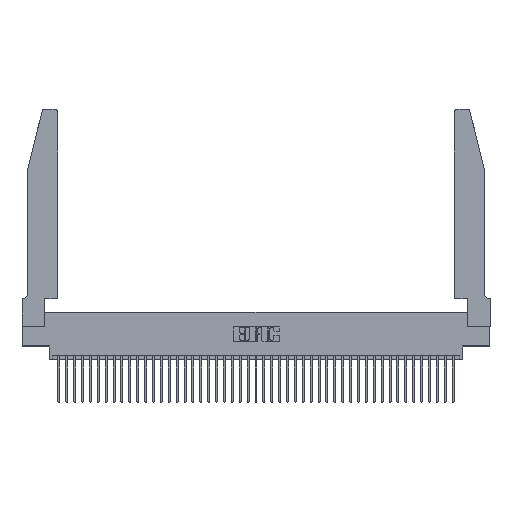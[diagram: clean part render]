
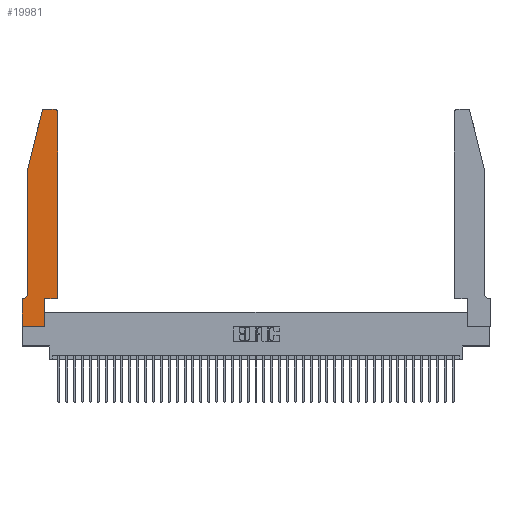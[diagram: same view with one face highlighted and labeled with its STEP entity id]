
A CAD part, top view. The second image highlights one B-rep face of the part: STEP entity #19981.
In plain terms, the highlighted planar face has unit normal (0, 0, 1).
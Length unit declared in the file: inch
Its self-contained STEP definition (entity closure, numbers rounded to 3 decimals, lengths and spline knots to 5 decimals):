
#165 = DIRECTION ( 'NONE',  ( 0., 1., 0. ) ) ;
#178 = CARTESIAN_POINT ( 'NONE',  ( 0.4505, 2.72, 0.37 ) ) ;
#245 = EDGE_CURVE ( 'NONE', #32430, #16549, #14913, .T. ) ;
#599 = ORIENTED_EDGE ( 'NONE', *, *, #18778, .T. ) ;
#636 = AXIS2_PLACEMENT_3D ( 'NONE', #8367, #5128, #24774 ) ;
#675 = DIRECTION ( 'NONE',  ( 1., 0., 0. ) ) ;
#732 = CARTESIAN_POINT ( 'NONE',  ( 0.0755, 2., 0.37 ) ) ;
#1567 = VECTOR ( 'NONE', #165, 39.37008 ) ;
#1759 = VERTEX_POINT ( 'NONE', #36868 ) ;
#1769 = EDGE_CURVE ( 'NONE', #6886, #20490, #16434, .T. ) ;
#1901 = DIRECTION ( 'NONE',  ( 0., -1., 0. ) ) ;
#2114 = DIRECTION ( 'NONE',  ( 1., 0., 0. ) ) ;
#3826 = CARTESIAN_POINT ( 'NONE',  ( 0.284, 2.75, 0.37 ) ) ;
#3864 = ORIENTED_EDGE ( 'NONE', *, *, #32552, .T. ) ;
#4105 = CARTESIAN_POINT ( 'NONE',  ( 0.2865, 0.35, 0.37 ) ) ;
#4147 = AXIS2_PLACEMENT_3D ( 'NONE', #11711, #27292, #17584 ) ;
#4201 = ORIENTED_EDGE ( 'NONE', *, *, #20687, .T. ) ;
#4270 = ORIENTED_EDGE ( 'NONE', *, *, #27838, .T. ) ;
#4411 = CIRCLE ( 'NONE', #636, 0.03 ) ;
#4865 = CARTESIAN_POINT ( 'NONE',  ( 0.4505, 0.35, 0.37 ) ) ;
#5128 = DIRECTION ( 'NONE',  ( 0., 0., 1. ) ) ;
#6208 = VECTOR ( 'NONE', #10135, 39.37008 ) ;
#6211 = LINE ( 'NONE', #732, #12591 ) ;
#6886 = VERTEX_POINT ( 'NONE', #26416 ) ;
#8097 = DIRECTION ( 'NONE',  ( 1., 0., 0. ) ) ;
#8367 = CARTESIAN_POINT ( 'NONE',  ( 0.4205, 2.72, 0.37 ) ) ;
#8573 = CARTESIAN_POINT ( 'NONE',  ( 0.0055, 0.35, 0.37 ) ) ;
#9091 = CIRCLE ( 'NONE', #4147, 0.03 ) ;
#10135 = DIRECTION ( 'NONE',  ( -1., 0., 0. ) ) ;
#10384 = ORIENTED_EDGE ( 'NONE', *, *, #33108, .T. ) ;
#10633 = VERTEX_POINT ( 'NONE', #16333 ) ;
#11314 = CARTESIAN_POINT ( 'NONE',  ( 0.2865, 0.35, 0.37 ) ) ;
#11371 = ORIENTED_EDGE ( 'NONE', *, *, #1769, .T. ) ;
#11610 = EDGE_CURVE ( 'NONE', #1759, #32430, #11691, .T. ) ;
#11691 = LINE ( 'NONE', #13510, #12738 ) ;
#11711 = CARTESIAN_POINT ( 'NONE',  ( 0.284, 2.72, 0.37 ) ) ;
#12343 = EDGE_CURVE ( 'NONE', #27216, #27855, #31111, .T. ) ;
#12591 = VECTOR ( 'NONE', #24200, 39.37008 ) ;
#12738 = VECTOR ( 'NONE', #1901, 39.37008 ) ;
#12824 = DIRECTION ( 'NONE',  ( 0., -1., 0. ) ) ;
#12882 = EDGE_CURVE ( 'NONE', #10633, #40637, #43618, .T. ) ;
#13162 = ORIENTED_EDGE ( 'NONE', *, *, #13765, .T. ) ;
#13510 = CARTESIAN_POINT ( 'NONE',  ( 0.0755, 2., 0.37 ) ) ;
#13765 = EDGE_CURVE ( 'NONE', #20490, #10633, #32407, .T. ) ;
#14526 = VERTEX_POINT ( 'NONE', #17843 ) ;
#14903 = ORIENTED_EDGE ( 'NONE', *, *, #12882, .T. ) ;
#14913 = CIRCLE ( 'NONE', #25679, 0.07 ) ;
#15534 = CARTESIAN_POINT ( 'NONE',  ( 0.4205, 2.75, 0.37 ) ) ;
#15649 = ORIENTED_EDGE ( 'NONE', *, *, #11610, .T. ) ;
#16333 = CARTESIAN_POINT ( 'NONE',  ( 0.2865, 0., 0.37 ) ) ;
#16434 = LINE ( 'NONE', #23338, #27982 ) ;
#16549 = VERTEX_POINT ( 'NONE', #8573 ) ;
#17463 = CARTESIAN_POINT ( 'NONE',  ( 0., 0., 0.37 ) ) ;
#17584 = DIRECTION ( 'NONE',  ( 1., 0., 0. ) ) ;
#17843 = CARTESIAN_POINT ( 'NONE',  ( 0.4505, 0.35, 0.37 ) ) ;
#17943 = CARTESIAN_POINT ( 'NONE',  ( 0.0055, 0.42, 0.37 ) ) ;
#18778 = EDGE_CURVE ( 'NONE', #40637, #14526, #30948, .T. ) ;
#19981 = ADVANCED_FACE ( 'NONE', ( #39925 ), #22115, .T. ) ;
#20103 = VERTEX_POINT ( 'NONE', #30167 ) ;
#20490 = VERTEX_POINT ( 'NONE', #17463 ) ;
#20687 = EDGE_CURVE ( 'NONE', #16549, #6886, #40031, .T. ) ;
#20914 = CARTESIAN_POINT ( 'NONE',  ( 0., 0.35, 0.37 ) ) ;
#21411 = ORIENTED_EDGE ( 'NONE', *, *, #12343, .T. ) ;
#22115 = PLANE ( 'NONE',  #25372 ) ;
#22797 = ORIENTED_EDGE ( 'NONE', *, *, #245, .T. ) ;
#23338 = CARTESIAN_POINT ( 'NONE',  ( 0., 0., 0.37 ) ) ;
#23391 = ORIENTED_EDGE ( 'NONE', *, *, #35457, .T. ) ;
#24200 = DIRECTION ( 'NONE',  ( -0.239, -0.971, 0. ) ) ;
#24774 = DIRECTION ( 'NONE',  ( 1., 0., 0. ) ) ;
#25309 = DIRECTION ( 'NONE',  ( 0., 0., 1. ) ) ;
#25372 = AXIS2_PLACEMENT_3D ( 'NONE', #20914, #25309, #675 ) ;
#25679 = AXIS2_PLACEMENT_3D ( 'NONE', #17943, #41259, #34586 ) ;
#25814 = VECTOR ( 'NONE', #34475, 39.37008 ) ;
#25973 = EDGE_LOOP ( 'NONE', ( #21411, #3864, #10384, #15649, #22797, #4201, #11371, #13162, #14903, #599, #4270, #23391 ) ) ;
#26029 = VERTEX_POINT ( 'NONE', #178 ) ;
#26416 = CARTESIAN_POINT ( 'NONE',  ( 0., 0.35, 0.37 ) ) ;
#27216 = VERTEX_POINT ( 'NONE', #15534 ) ;
#27292 = DIRECTION ( 'NONE',  ( 0., 0., 1. ) ) ;
#27838 = EDGE_CURVE ( 'NONE', #14526, #26029, #41746, .T. ) ;
#27855 = VERTEX_POINT ( 'NONE', #3826 ) ;
#27982 = VECTOR ( 'NONE', #12824, 39.37008 ) ;
#29969 = CARTESIAN_POINT ( 'NONE',  ( 0.0755, 0.42, 0.37 ) ) ;
#30167 = CARTESIAN_POINT ( 'NONE',  ( 0.25487, 2.72718, 0.37 ) ) ;
#30249 = VECTOR ( 'NONE', #2114, 39.37008 ) ;
#30316 = CARTESIAN_POINT ( 'NONE',  ( 0.0755, 0.35, 0.37 ) ) ;
#30816 = DIRECTION ( 'NONE',  ( 0., 1., 0. ) ) ;
#30948 = LINE ( 'NONE', #4865, #38356 ) ;
#31111 = LINE ( 'NONE', #41440, #25814 ) ;
#31800 = CARTESIAN_POINT ( 'NONE',  ( 0., 0., 0.37 ) ) ;
#32407 = LINE ( 'NONE', #31800, #30249 ) ;
#32430 = VERTEX_POINT ( 'NONE', #29969 ) ;
#32552 = EDGE_CURVE ( 'NONE', #27855, #20103, #9091, .T. ) ;
#33108 = EDGE_CURVE ( 'NONE', #20103, #1759, #6211, .T. ) ;
#34475 = DIRECTION ( 'NONE',  ( -1., 0., 0. ) ) ;
#34579 = VECTOR ( 'NONE', #30816, 39.37008 ) ;
#34586 = DIRECTION ( 'NONE',  ( -1., 0., 0. ) ) ;
#35457 = EDGE_CURVE ( 'NONE', #26029, #27216, #4411, .T. ) ;
#36868 = CARTESIAN_POINT ( 'NONE',  ( 0.0755, 2., 0.37 ) ) ;
#38356 = VECTOR ( 'NONE', #8097, 39.37008 ) ;
#39925 = FACE_OUTER_BOUND ( 'NONE', #25973, .T. ) ;
#40031 = LINE ( 'NONE', #30316, #6208 ) ;
#40637 = VERTEX_POINT ( 'NONE', #11314 ) ;
#41162 = CARTESIAN_POINT ( 'NONE',  ( 0.4505, 0.35, 0.37 ) ) ;
#41259 = DIRECTION ( 'NONE',  ( 0., 0., -1. ) ) ;
#41440 = CARTESIAN_POINT ( 'NONE',  ( 0.2605, 2.75, 0.37 ) ) ;
#41746 = LINE ( 'NONE', #41162, #1567 ) ;
#43618 = LINE ( 'NONE', #4105, #34579 ) ;
